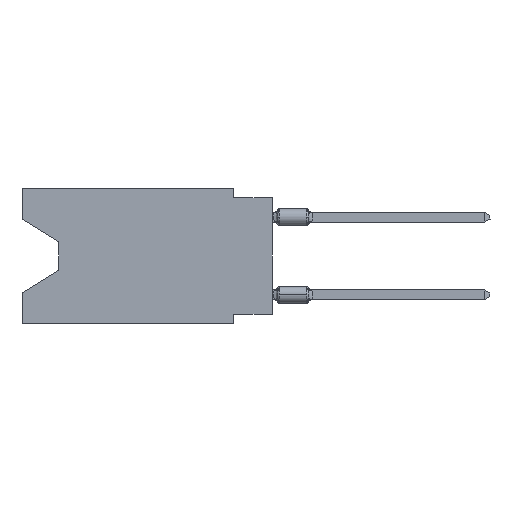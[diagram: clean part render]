
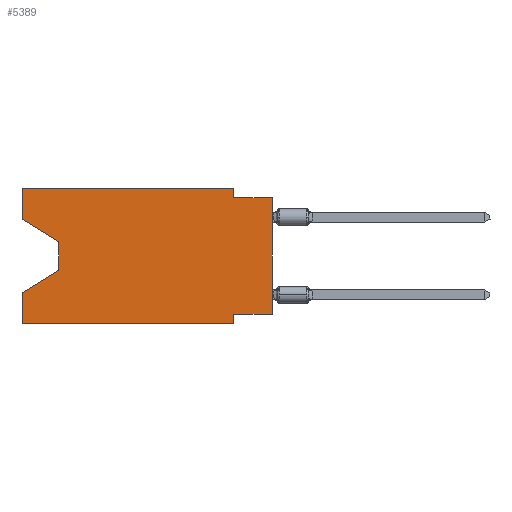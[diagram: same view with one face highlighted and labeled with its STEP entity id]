
A CAD part, left-side view. The second image highlights one B-rep face of the part: STEP entity #5389.
In plain terms, the highlighted planar face has unit normal (-1, 0, 0).
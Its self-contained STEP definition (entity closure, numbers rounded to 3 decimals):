
#1 = ORIENTED_EDGE ( 'NONE', *, *, #13189, .T. ) ;
#135 = CARTESIAN_POINT ( 'NONE',  ( 0., 16.383, 0. ) ) ;
#491 = CARTESIAN_POINT ( 'NONE',  ( 0., 2.54, 0. ) ) ;
#1059 = DIRECTION ( 'NONE',  ( 0., -1., 0. ) ) ;
#1270 = ORIENTED_EDGE ( 'NONE', *, *, #6716, .T. ) ;
#2269 = VERTEX_POINT ( 'NONE', #14251 ) ;
#2561 = CARTESIAN_POINT ( 'NONE',  ( 0., 2.54, -8.255 ) ) ;
#2997 = EDGE_CURVE ( 'NONE', #7499, #32385, #4560, .T. ) ;
#3803 = AXIS2_PLACEMENT_3D ( 'NONE', #10345, #21720, #4819 ) ;
#4034 = CARTESIAN_POINT ( 'NONE',  ( 0., 16.383, -2.038 ) ) ;
#4560 = LINE ( 'NONE', #29650, #6593 ) ;
#4819 = DIRECTION ( 'NONE',  ( 0., 0., -1. ) ) ;
#5003 = PLANE ( 'NONE',  #3803 ) ;
#5339 = EDGE_CURVE ( 'NONE', #18247, #33723, #9640, .T. ) ;
#5389 = ADVANCED_FACE ( 'NONE', ( #24393 ), #5003, .F. ) ;
#6593 = VECTOR ( 'NONE', #16143, 1000. ) ;
#6716 = EDGE_CURVE ( 'NONE', #17527, #30879, #16929, .T. ) ;
#7475 = VECTOR ( 'NONE', #1059, 1000. ) ;
#7488 = ORIENTED_EDGE ( 'NONE', *, *, #12093, .T. ) ;
#7499 = VERTEX_POINT ( 'NONE', #24647 ) ;
#7552 = VECTOR ( 'NONE', #11342, 1000. ) ;
#7970 = EDGE_CURVE ( 'NONE', #24660, #32385, #27565, .T. ) ;
#8904 = DIRECTION ( 'NONE',  ( 0., 0.855, -0.519 ) ) ;
#8954 = CARTESIAN_POINT ( 'NONE',  ( 0., 16.383, 0. ) ) ;
#9620 = EDGE_CURVE ( 'NONE', #13927, #11985, #10471, .T. ) ;
#9640 = LINE ( 'NONE', #20498, #33893 ) ;
#9775 = EDGE_CURVE ( 'NONE', #11985, #24660, #22370, .T. ) ;
#10345 = CARTESIAN_POINT ( 'NONE',  ( 0., 16.383, 0. ) ) ;
#10471 = LINE ( 'NONE', #135, #26894 ) ;
#10966 = EDGE_LOOP ( 'NONE', ( #7488, #1, #1270, #13767, #34510, #16240, #35028, #17817, #26542, #11784, #19398, #29935 ) ) ;
#11232 = CARTESIAN_POINT ( 'NONE',  ( 0., 13.97, -3.505 ) ) ;
#11342 = DIRECTION ( 'NONE',  ( 0., 0., -1. ) ) ;
#11660 = VECTOR ( 'NONE', #27985, 1000. ) ;
#11719 = VERTEX_POINT ( 'NONE', #2561 ) ;
#11784 = ORIENTED_EDGE ( 'NONE', *, *, #9775, .F. ) ;
#11877 = CARTESIAN_POINT ( 'NONE',  ( 0., 16.383, -8.89 ) ) ;
#11985 = VERTEX_POINT ( 'NONE', #24694 ) ;
#12093 = EDGE_CURVE ( 'NONE', #28358, #2269, #20597, .T. ) ;
#12324 = VECTOR ( 'NONE', #18492, 1000. ) ;
#12831 = CARTESIAN_POINT ( 'NONE',  ( 0., 0., -8.255 ) ) ;
#13189 = EDGE_CURVE ( 'NONE', #2269, #17527, #21731, .T. ) ;
#13767 = ORIENTED_EDGE ( 'NONE', *, *, #20564, .F. ) ;
#13927 = VERTEX_POINT ( 'NONE', #8954 ) ;
#14251 = CARTESIAN_POINT ( 'NONE',  ( 0., 13.97, -3.505 ) ) ;
#14351 = CARTESIAN_POINT ( 'NONE',  ( 0., 16.383, 0. ) ) ;
#14387 = CARTESIAN_POINT ( 'NONE',  ( 0., 2.54, -0.635 ) ) ;
#14704 = DIRECTION ( 'NONE',  ( 0., 0., 1. ) ) ;
#15687 = DIRECTION ( 'NONE',  ( 0., 1., 0. ) ) ;
#16143 = DIRECTION ( 'NONE',  ( 0., 0., 1. ) ) ;
#16240 = ORIENTED_EDGE ( 'NONE', *, *, #27042, .F. ) ;
#16929 = LINE ( 'NONE', #19596, #26144 ) ;
#17031 = LINE ( 'NONE', #14351, #27680 ) ;
#17150 = LINE ( 'NONE', #19645, #11660 ) ;
#17247 = CARTESIAN_POINT ( 'NONE',  ( 0., 0., -0.635 ) ) ;
#17527 = VERTEX_POINT ( 'NONE', #20496 ) ;
#17768 = EDGE_CURVE ( 'NONE', #7499, #11719, #31696, .T. ) ;
#17817 = ORIENTED_EDGE ( 'NONE', *, *, #2997, .T. ) ;
#17827 = DIRECTION ( 'NONE',  ( 0., -1., 0. ) ) ;
#18247 = VERTEX_POINT ( 'NONE', #11877 ) ;
#18492 = DIRECTION ( 'NONE',  ( 0., 0., -1. ) ) ;
#18907 = LINE ( 'NONE', #34498, #12324 ) ;
#19398 = ORIENTED_EDGE ( 'NONE', *, *, #9620, .F. ) ;
#19596 = CARTESIAN_POINT ( 'NONE',  ( 0., 13.97, -5.385 ) ) ;
#19603 = VECTOR ( 'NONE', #29748, 1000. ) ;
#19645 = CARTESIAN_POINT ( 'NONE',  ( 0., 16.383, 0. ) ) ;
#20496 = CARTESIAN_POINT ( 'NONE',  ( 0., 13.97, -5.385 ) ) ;
#20498 = CARTESIAN_POINT ( 'NONE',  ( 0., 16.383, -8.89 ) ) ;
#20564 = EDGE_CURVE ( 'NONE', #18247, #30879, #17150, .T. ) ;
#20597 = LINE ( 'NONE', #4034, #32039 ) ;
#21720 = DIRECTION ( 'NONE',  ( 1., 0., 0. ) ) ;
#21731 = LINE ( 'NONE', #11232, #19603 ) ;
#21845 = DIRECTION ( 'NONE',  ( 0., -1., 0. ) ) ;
#22370 = LINE ( 'NONE', #491, #7552 ) ;
#22654 = VECTOR ( 'NONE', #15687, 1000. ) ;
#24393 = FACE_OUTER_BOUND ( 'NONE', #10966, .T. ) ;
#24647 = CARTESIAN_POINT ( 'NONE',  ( 0., 0., -8.255 ) ) ;
#24660 = VERTEX_POINT ( 'NONE', #14387 ) ;
#24694 = CARTESIAN_POINT ( 'NONE',  ( 0., 2.54, 0. ) ) ;
#24756 = CARTESIAN_POINT ( 'NONE',  ( 0., 0., -0.635 ) ) ;
#26144 = VECTOR ( 'NONE', #8904, 1000. ) ;
#26269 = DIRECTION ( 'NONE',  ( 0., -0.855, -0.519 ) ) ;
#26399 = CARTESIAN_POINT ( 'NONE',  ( 0., 16.383, -6.852 ) ) ;
#26542 = ORIENTED_EDGE ( 'NONE', *, *, #7970, .F. ) ;
#26894 = VECTOR ( 'NONE', #21845, 1000. ) ;
#27042 = EDGE_CURVE ( 'NONE', #11719, #33723, #18907, .T. ) ;
#27565 = LINE ( 'NONE', #17247, #7475 ) ;
#27680 = VECTOR ( 'NONE', #14704, 1000. ) ;
#27985 = DIRECTION ( 'NONE',  ( 0., 0., 1. ) ) ;
#28358 = VERTEX_POINT ( 'NONE', #33341 ) ;
#28484 = CARTESIAN_POINT ( 'NONE',  ( 0., 2.54, -8.89 ) ) ;
#29650 = CARTESIAN_POINT ( 'NONE',  ( 0., 0., 0. ) ) ;
#29748 = DIRECTION ( 'NONE',  ( 0., 0., -1. ) ) ;
#29935 = ORIENTED_EDGE ( 'NONE', *, *, #31502, .F. ) ;
#30879 = VERTEX_POINT ( 'NONE', #26399 ) ;
#31502 = EDGE_CURVE ( 'NONE', #28358, #13927, #17031, .T. ) ;
#31696 = LINE ( 'NONE', #12831, #22654 ) ;
#32039 = VECTOR ( 'NONE', #26269, 1000. ) ;
#32385 = VERTEX_POINT ( 'NONE', #24756 ) ;
#33341 = CARTESIAN_POINT ( 'NONE',  ( 0., 16.383, -2.038 ) ) ;
#33723 = VERTEX_POINT ( 'NONE', #28484 ) ;
#33893 = VECTOR ( 'NONE', #17827, 1000. ) ;
#34498 = CARTESIAN_POINT ( 'NONE',  ( 0., 2.54, -8.89 ) ) ;
#34510 = ORIENTED_EDGE ( 'NONE', *, *, #5339, .T. ) ;
#35028 = ORIENTED_EDGE ( 'NONE', *, *, #17768, .F. ) ;
